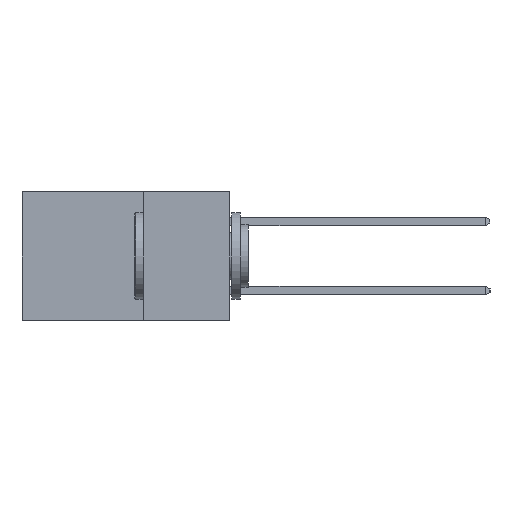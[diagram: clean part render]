
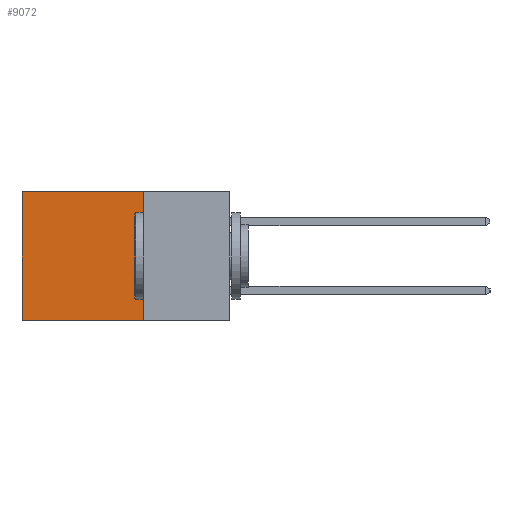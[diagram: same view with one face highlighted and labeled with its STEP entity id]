
A CAD part, left-side view. The second image highlights one B-rep face of the part: STEP entity #9072.
In plain terms, the highlighted planar face has unit normal (-1, 0, 0).
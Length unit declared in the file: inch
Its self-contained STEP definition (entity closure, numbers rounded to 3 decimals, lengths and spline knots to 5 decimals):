
#357 = EDGE_LOOP ( 'NONE', ( #4860, #13627, #6121, #11718 ) ) ;
#1673 = LINE ( 'NONE', #9606, #13076 ) ;
#1772 = VECTOR ( 'NONE', #11826, 39.37008 ) ;
#2139 = VERTEX_POINT ( 'NONE', #11362 ) ;
#2216 = VERTEX_POINT ( 'NONE', #9408 ) ;
#3289 = EDGE_CURVE ( 'NONE', #3896, #2139, #8905, .T. ) ;
#3799 = EDGE_CURVE ( 'NONE', #2216, #6435, #13477, .T. ) ;
#3896 = VERTEX_POINT ( 'NONE', #7543 ) ;
#4537 = FACE_OUTER_BOUND ( 'NONE', #357, .T. ) ;
#4860 = ORIENTED_EDGE ( 'NONE', *, *, #7721, .T. ) ;
#5444 = AXIS2_PLACEMENT_3D ( 'NONE', #13706, #13102, #13016 ) ;
#6089 = CARTESIAN_POINT ( 'NONE',  ( 0.2615, 0.25, -0.37 ) ) ;
#6121 = ORIENTED_EDGE ( 'NONE', *, *, #12727, .F. ) ;
#6189 = DIRECTION ( 'NONE',  ( 0., 1., 0. ) ) ;
#6435 = VERTEX_POINT ( 'NONE', #10093 ) ;
#7543 = CARTESIAN_POINT ( 'NONE',  ( 0.2615, 0.25, -0.37 ) ) ;
#7721 = EDGE_CURVE ( 'NONE', #6435, #2139, #1673, .T. ) ;
#7841 = CARTESIAN_POINT ( 'NONE',  ( 0.2615, 0.25, 0. ) ) ;
#8776 = DIRECTION ( 'NONE',  ( 0., 0., -1. ) ) ;
#8905 = LINE ( 'NONE', #6089, #11705 ) ;
#9072 = ADVANCED_FACE ( 'NONE', ( #4537 ), #13166, .F. ) ;
#9384 = LINE ( 'NONE', #12438, #11522 ) ;
#9408 = CARTESIAN_POINT ( 'NONE',  ( 0.2615, 0.25, 0. ) ) ;
#9606 = CARTESIAN_POINT ( 'NONE',  ( 0.2615, 0.6, -0.37 ) ) ;
#10093 = CARTESIAN_POINT ( 'NONE',  ( 0.2615, 0.6, 0. ) ) ;
#11362 = CARTESIAN_POINT ( 'NONE',  ( 0.2615, 0.6, -0.37 ) ) ;
#11522 = VECTOR ( 'NONE', #12502, 39.37008 ) ;
#11705 = VECTOR ( 'NONE', #6189, 39.37008 ) ;
#11718 = ORIENTED_EDGE ( 'NONE', *, *, #3799, .T. ) ;
#11826 = DIRECTION ( 'NONE',  ( 0., 1., 0. ) ) ;
#12438 = CARTESIAN_POINT ( 'NONE',  ( 0.2615, 0.25, -0.37 ) ) ;
#12502 = DIRECTION ( 'NONE',  ( 0., 0., -1. ) ) ;
#12727 = EDGE_CURVE ( 'NONE', #2216, #3896, #9384, .T. ) ;
#13016 = DIRECTION ( 'NONE',  ( 0., 0., -1. ) ) ;
#13076 = VECTOR ( 'NONE', #8776, 39.37008 ) ;
#13102 = DIRECTION ( 'NONE',  ( 1., 0., 0. ) ) ;
#13166 = PLANE ( 'NONE',  #5444 ) ;
#13477 = LINE ( 'NONE', #7841, #1772 ) ;
#13627 = ORIENTED_EDGE ( 'NONE', *, *, #3289, .F. ) ;
#13706 = CARTESIAN_POINT ( 'NONE',  ( 0.2615, 0.25, -0.37 ) ) ;
